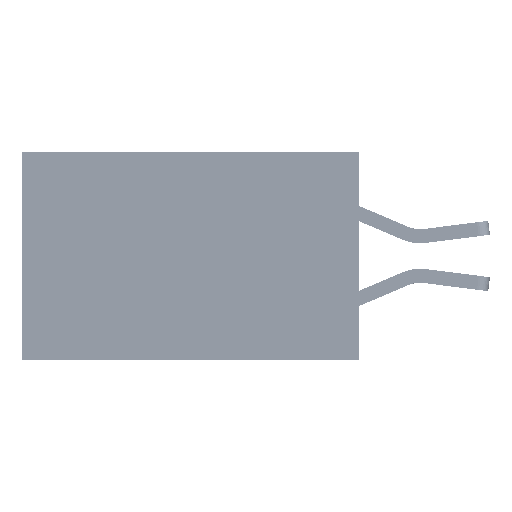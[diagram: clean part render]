
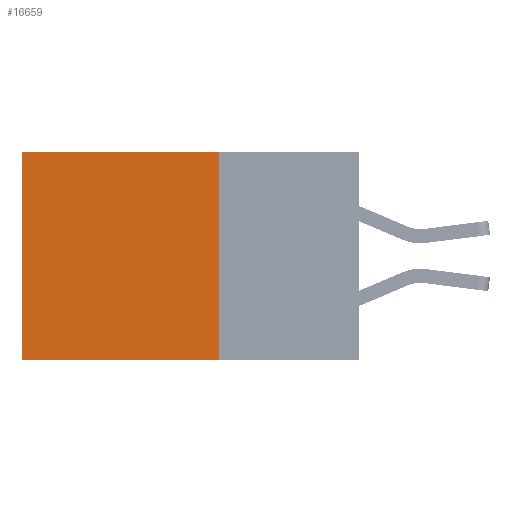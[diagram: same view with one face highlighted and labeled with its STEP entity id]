
A CAD part, left-side view. The second image highlights one B-rep face of the part: STEP entity #16659.
In plain terms, the highlighted planar face has unit normal (-1, 0, 0).
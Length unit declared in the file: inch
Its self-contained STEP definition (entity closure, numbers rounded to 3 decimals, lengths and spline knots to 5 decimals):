
#1156 = CARTESIAN_POINT ( 'NONE',  ( 0.2875, 0.6, 0. ) ) ;
#3668 = DIRECTION ( 'NONE',  ( 0., 0., -1. ) ) ;
#4293 = CARTESIAN_POINT ( 'NONE',  ( 0.2875, 0.25, -0.37 ) ) ;
#7280 = DIRECTION ( 'NONE',  ( 0., 0., -1. ) ) ;
#8830 = VERTEX_POINT ( 'NONE', #24516 ) ;
#10816 = PLANE ( 'NONE',  #16441 ) ;
#16441 = AXIS2_PLACEMENT_3D ( 'NONE', #38071, #27560, #3668 ) ;
#16659 = ADVANCED_FACE ( 'NONE', ( #37839 ), #10816, .F. ) ;
#18256 = EDGE_CURVE ( 'NONE', #37433, #32179, #24245, .T. ) ;
#18659 = CARTESIAN_POINT ( 'NONE',  ( 0.2875, 0.6, 0. ) ) ;
#19369 = ORIENTED_EDGE ( 'NONE', *, *, #43774, .T. ) ;
#19509 = DIRECTION ( 'NONE',  ( 0., 1., 0. ) ) ;
#19556 = CARTESIAN_POINT ( 'NONE',  ( 0.2875, 0.25, 0. ) ) ;
#21474 = DIRECTION ( 'NONE',  ( 0., 0., -1. ) ) ;
#21899 = VECTOR ( 'NONE', #25307, 39.37008 ) ;
#21954 = CARTESIAN_POINT ( 'NONE',  ( 0.2875, 0.25, 0. ) ) ;
#24245 = LINE ( 'NONE', #38102, #26516 ) ;
#24516 = CARTESIAN_POINT ( 'NONE',  ( 0.2875, 0.6, -0.37 ) ) ;
#24563 = VECTOR ( 'NONE', #21474, 39.37008 ) ;
#25307 = DIRECTION ( 'NONE',  ( 0., 1., 0. ) ) ;
#25767 = CARTESIAN_POINT ( 'NONE',  ( 0.2875, 0.25, -0.37 ) ) ;
#26140 = VERTEX_POINT ( 'NONE', #18659 ) ;
#26516 = VECTOR ( 'NONE', #7280, 39.37008 ) ;
#27560 = DIRECTION ( 'NONE',  ( 1., 0., 0. ) ) ;
#31590 = LINE ( 'NONE', #21954, #21899 ) ;
#32179 = VERTEX_POINT ( 'NONE', #4293 ) ;
#32302 = ORIENTED_EDGE ( 'NONE', *, *, #36732, .T. ) ;
#33382 = ORIENTED_EDGE ( 'NONE', *, *, #39622, .F. ) ;
#36732 = EDGE_CURVE ( 'NONE', #26140, #8830, #41822, .T. ) ;
#37433 = VERTEX_POINT ( 'NONE', #19556 ) ;
#37839 = FACE_OUTER_BOUND ( 'NONE', #38935, .T. ) ;
#38071 = CARTESIAN_POINT ( 'NONE',  ( 0.2875, 0.25, 0. ) ) ;
#38102 = CARTESIAN_POINT ( 'NONE',  ( 0.2875, 0.25, 0. ) ) ;
#38369 = LINE ( 'NONE', #25767, #39697 ) ;
#38935 = EDGE_LOOP ( 'NONE', ( #32302, #33382, #43349, #19369 ) ) ;
#39622 = EDGE_CURVE ( 'NONE', #32179, #8830, #38369, .T. ) ;
#39697 = VECTOR ( 'NONE', #19509, 39.37008 ) ;
#41822 = LINE ( 'NONE', #1156, #24563 ) ;
#43349 = ORIENTED_EDGE ( 'NONE', *, *, #18256, .F. ) ;
#43774 = EDGE_CURVE ( 'NONE', #37433, #26140, #31590, .T. ) ;
